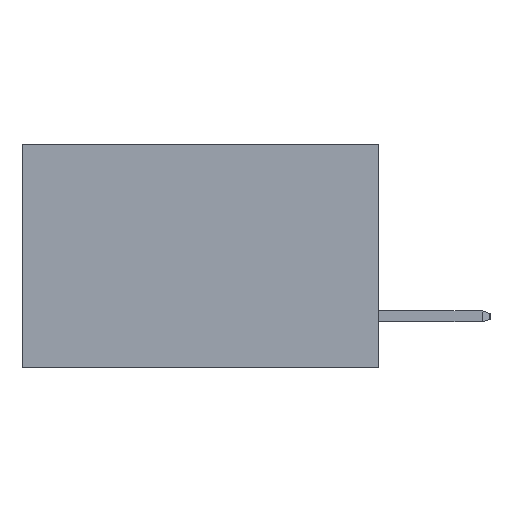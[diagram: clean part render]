
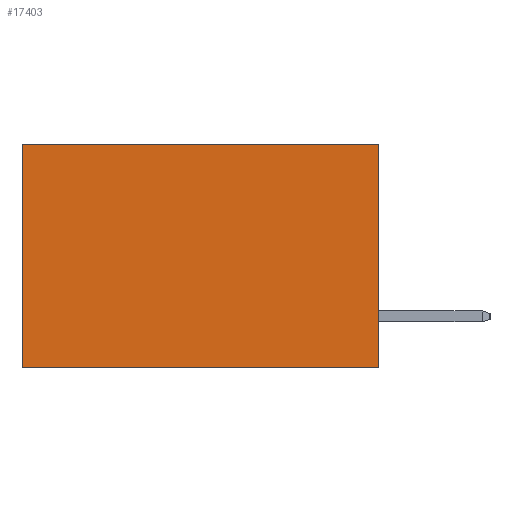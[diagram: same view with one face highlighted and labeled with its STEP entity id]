
A CAD part, left-side view. The second image highlights one B-rep face of the part: STEP entity #17403.
In plain terms, the highlighted planar face has unit normal (-1, 0, 0).
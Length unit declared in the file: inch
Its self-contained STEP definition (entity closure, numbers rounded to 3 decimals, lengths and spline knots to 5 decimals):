
#278 = CARTESIAN_POINT ( 'NONE',  ( 0.277, 0., 0. ) ) ;
#372 = CARTESIAN_POINT ( 'NONE',  ( 0.277, 0., -0.37 ) ) ;
#554 = VERTEX_POINT ( 'NONE', #9690 ) ;
#854 = VERTEX_POINT ( 'NONE', #17478 ) ;
#908 = CARTESIAN_POINT ( 'NONE',  ( 0.277, 0.59, -0.37 ) ) ;
#1093 = DIRECTION ( 'NONE',  ( 0., 1., 0. ) ) ;
#1362 = LINE ( 'NONE', #372, #18929 ) ;
#1572 = VECTOR ( 'NONE', #1093, 39.37008 ) ;
#1676 = ORIENTED_EDGE ( 'NONE', *, *, #4569, .T. ) ;
#2068 = LINE ( 'NONE', #908, #11168 ) ;
#2459 = DIRECTION ( 'NONE',  ( 0., 0., -1. ) ) ;
#3922 = CARTESIAN_POINT ( 'NONE',  ( 0.277, 0., 0. ) ) ;
#4569 = EDGE_CURVE ( 'NONE', #9874, #16639, #13932, .T. ) ;
#4905 = CARTESIAN_POINT ( 'NONE',  ( 0.277, 0., -0.37 ) ) ;
#7043 = ORIENTED_EDGE ( 'NONE', *, *, #19743, .T. ) ;
#8334 = DIRECTION ( 'NONE',  ( 0., 0., -1. ) ) ;
#8831 = FACE_OUTER_BOUND ( 'NONE', #17784, .T. ) ;
#9426 = EDGE_CURVE ( 'NONE', #554, #854, #10174, .T. ) ;
#9690 = CARTESIAN_POINT ( 'NONE',  ( 0.277, 0., -0.37 ) ) ;
#9874 = VERTEX_POINT ( 'NONE', #3922 ) ;
#10174 = LINE ( 'NONE', #21427, #1572 ) ;
#11168 = VECTOR ( 'NONE', #2459, 39.37008 ) ;
#12689 = ORIENTED_EDGE ( 'NONE', *, *, #16262, .F. ) ;
#12863 = VECTOR ( 'NONE', #21331, 39.37008 ) ;
#13266 = CARTESIAN_POINT ( 'NONE',  ( 0.277, 0.59, 0. ) ) ;
#13932 = LINE ( 'NONE', #278, #12863 ) ;
#15153 = PLANE ( 'NONE',  #15970 ) ;
#15970 = AXIS2_PLACEMENT_3D ( 'NONE', #4905, #18478, #8334 ) ;
#16262 = EDGE_CURVE ( 'NONE', #9874, #554, #1362, .T. ) ;
#16639 = VERTEX_POINT ( 'NONE', #13266 ) ;
#17349 = DIRECTION ( 'NONE',  ( 0., 0., -1. ) ) ;
#17403 = ADVANCED_FACE ( 'NONE', ( #8831 ), #15153, .F. ) ;
#17478 = CARTESIAN_POINT ( 'NONE',  ( 0.277, 0.59, -0.37 ) ) ;
#17784 = EDGE_LOOP ( 'NONE', ( #7043, #20554, #12689, #1676 ) ) ;
#18478 = DIRECTION ( 'NONE',  ( 1., 0., 0. ) ) ;
#18929 = VECTOR ( 'NONE', #17349, 39.37008 ) ;
#19743 = EDGE_CURVE ( 'NONE', #16639, #854, #2068, .T. ) ;
#20554 = ORIENTED_EDGE ( 'NONE', *, *, #9426, .F. ) ;
#21331 = DIRECTION ( 'NONE',  ( 0., 1., 0. ) ) ;
#21427 = CARTESIAN_POINT ( 'NONE',  ( 0.277, 0., -0.37 ) ) ;
